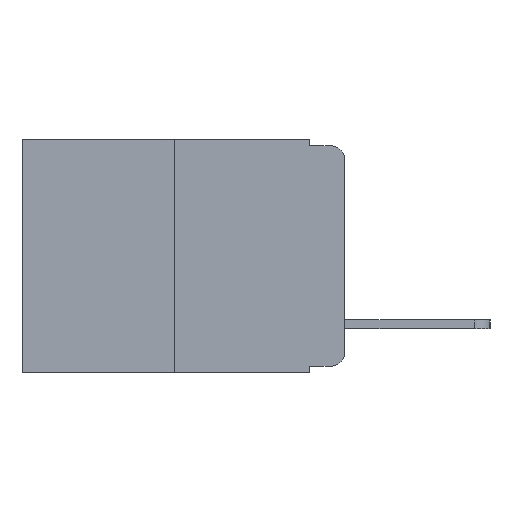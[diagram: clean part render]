
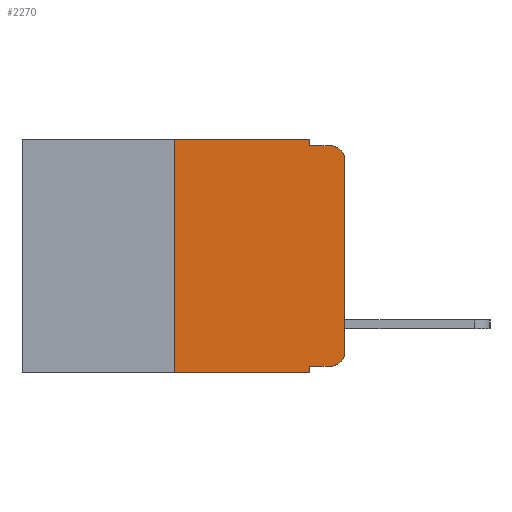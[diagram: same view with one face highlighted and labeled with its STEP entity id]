
A CAD part, left-side view. The second image highlights one B-rep face of the part: STEP entity #2270.
In plain terms, the highlighted planar face has unit normal (-1, 0, 0).
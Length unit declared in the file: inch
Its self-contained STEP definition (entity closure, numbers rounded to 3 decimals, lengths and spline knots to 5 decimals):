
#730 = AXIS2_PLACEMENT_3D ( 'NONE', #4865, #1582, #7941 ) ;
#749 = CARTESIAN_POINT ( 'NONE',  ( 0., 0., -0.03 ) ) ;
#792 = ORIENTED_EDGE ( 'NONE', *, *, #5768, .T. ) ;
#857 = CARTESIAN_POINT ( 'NONE',  ( 0., 0.051, -0.333 ) ) ;
#1050 = ORIENTED_EDGE ( 'NONE', *, *, #5008, .T. ) ;
#1187 = LINE ( 'NONE', #3296, #5474 ) ;
#1582 = DIRECTION ( 'NONE',  ( -1., 0., 0. ) ) ;
#1626 = CARTESIAN_POINT ( 'NONE',  ( 0., 0.25, 0. ) ) ;
#1706 = DIRECTION ( 'NONE',  ( 0., 0., -1. ) ) ;
#1768 = DIRECTION ( 'NONE',  ( 0., 0., -1. ) ) ;
#1894 = CIRCLE ( 'NONE', #2462, 0.02 ) ;
#1895 = CARTESIAN_POINT ( 'NONE',  ( 0., 0.25, 0. ) ) ;
#2013 = ORIENTED_EDGE ( 'NONE', *, *, #5486, .F. ) ;
#2041 = CARTESIAN_POINT ( 'NONE',  ( 0., 0.051, -0.01 ) ) ;
#2056 = VECTOR ( 'NONE', #8655, 39.37008 ) ;
#2193 = VERTEX_POINT ( 'NONE', #9770 ) ;
#2208 = VECTOR ( 'NONE', #6875, 39.37008 ) ;
#2270 = ADVANCED_FACE ( 'NONE', ( #4684 ), #4463, .F. ) ;
#2276 = VERTEX_POINT ( 'NONE', #5153 ) ;
#2317 = ORIENTED_EDGE ( 'NONE', *, *, #5647, .F. ) ;
#2462 = AXIS2_PLACEMENT_3D ( 'NONE', #5428, #5593, #1768 ) ;
#2519 = LINE ( 'NONE', #9685, #8420 ) ;
#2572 = DIRECTION ( 'NONE',  ( 0., -1., 0. ) ) ;
#2662 = EDGE_CURVE ( 'NONE', #4297, #4433, #1187, .T. ) ;
#2743 = CARTESIAN_POINT ( 'NONE',  ( 0., 0., 0. ) ) ;
#2974 = VECTOR ( 'NONE', #2572, 39.37008 ) ;
#3042 = DIRECTION ( 'NONE',  ( 0., 0., 1. ) ) ;
#3130 = CIRCLE ( 'NONE', #730, 0.02 ) ;
#3169 = AXIS2_PLACEMENT_3D ( 'NONE', #5853, #4576, #4569 ) ;
#3296 = CARTESIAN_POINT ( 'NONE',  ( 0., 0.473, -0.343 ) ) ;
#3309 = DIRECTION ( 'NONE',  ( 0., -1., 0. ) ) ;
#3364 = CARTESIAN_POINT ( 'NONE',  ( 0., 0.051, -0.333 ) ) ;
#3381 = ORIENTED_EDGE ( 'NONE', *, *, #5251, .F. ) ;
#4239 = VERTEX_POINT ( 'NONE', #1895 ) ;
#4297 = VERTEX_POINT ( 'NONE', #7303 ) ;
#4299 = LINE ( 'NONE', #6160, #6185 ) ;
#4433 = VERTEX_POINT ( 'NONE', #5621 ) ;
#4463 = PLANE ( 'NONE',  #3169 ) ;
#4569 = DIRECTION ( 'NONE',  ( 0., 0., -1. ) ) ;
#4576 = DIRECTION ( 'NONE',  ( 1., 0., 0. ) ) ;
#4588 = LINE ( 'NONE', #3364, #2208 ) ;
#4623 = CARTESIAN_POINT ( 'NONE',  ( 0., 0.02, -0.333 ) ) ;
#4684 = FACE_OUTER_BOUND ( 'NONE', #5697, .T. ) ;
#4700 = LINE ( 'NONE', #9311, #2056 ) ;
#4778 = DIRECTION ( 'NONE',  ( 0., -1., 0. ) ) ;
#4865 = CARTESIAN_POINT ( 'NONE',  ( 0., 0.02, -0.03 ) ) ;
#5008 = EDGE_CURVE ( 'NONE', #2276, #9101, #6620, .T. ) ;
#5024 = ORIENTED_EDGE ( 'NONE', *, *, #5137, .T. ) ;
#5086 = VERTEX_POINT ( 'NONE', #857 ) ;
#5137 = EDGE_CURVE ( 'NONE', #9101, #9544, #3130, .T. ) ;
#5153 = CARTESIAN_POINT ( 'NONE',  ( 0., 0., -0.313 ) ) ;
#5251 = EDGE_CURVE ( 'NONE', #5674, #9544, #7285, .T. ) ;
#5295 = LINE ( 'NONE', #1626, #6934 ) ;
#5322 = EDGE_CURVE ( 'NONE', #2193, #5674, #4700, .T. ) ;
#5323 = CARTESIAN_POINT ( 'NONE',  ( 0., 0.051, -0.01 ) ) ;
#5428 = CARTESIAN_POINT ( 'NONE',  ( 0., 0.02, -0.313 ) ) ;
#5474 = VECTOR ( 'NONE', #3309, 39.37008 ) ;
#5486 = EDGE_CURVE ( 'NONE', #4297, #4239, #5295, .T. ) ;
#5593 = DIRECTION ( 'NONE',  ( -1., 0., 0. ) ) ;
#5621 = CARTESIAN_POINT ( 'NONE',  ( 0., 0.051, -0.343 ) ) ;
#5647 = EDGE_CURVE ( 'NONE', #5086, #4433, #2519, .T. ) ;
#5674 = VERTEX_POINT ( 'NONE', #5323 ) ;
#5697 = EDGE_LOOP ( 'NONE', ( #1050, #5024, #3381, #7355, #5888, #2013, #8284, #2317, #8948, #792 ) ) ;
#5703 = EDGE_CURVE ( 'NONE', #5086, #5995, #4588, .T. ) ;
#5768 = EDGE_CURVE ( 'NONE', #5995, #2276, #1894, .T. ) ;
#5853 = CARTESIAN_POINT ( 'NONE',  ( 0., 0.473, 0. ) ) ;
#5888 = ORIENTED_EDGE ( 'NONE', *, *, #9551, .F. ) ;
#5995 = VERTEX_POINT ( 'NONE', #4623 ) ;
#6160 = CARTESIAN_POINT ( 'NONE',  ( 0., 0.473, 0. ) ) ;
#6185 = VECTOR ( 'NONE', #4778, 39.37008 ) ;
#6620 = LINE ( 'NONE', #2743, #9951 ) ;
#6875 = DIRECTION ( 'NONE',  ( 0., -1., 0. ) ) ;
#6934 = VECTOR ( 'NONE', #3042, 39.37008 ) ;
#7285 = LINE ( 'NONE', #2041, #2974 ) ;
#7303 = CARTESIAN_POINT ( 'NONE',  ( 0., 0.25, -0.343 ) ) ;
#7355 = ORIENTED_EDGE ( 'NONE', *, *, #5322, .F. ) ;
#7941 = DIRECTION ( 'NONE',  ( 0., 0., -1. ) ) ;
#8284 = ORIENTED_EDGE ( 'NONE', *, *, #2662, .T. ) ;
#8420 = VECTOR ( 'NONE', #1706, 39.37008 ) ;
#8655 = DIRECTION ( 'NONE',  ( 0., 0., -1. ) ) ;
#8732 = DIRECTION ( 'NONE',  ( 0., 0., 1. ) ) ;
#8948 = ORIENTED_EDGE ( 'NONE', *, *, #5703, .T. ) ;
#9101 = VERTEX_POINT ( 'NONE', #749 ) ;
#9311 = CARTESIAN_POINT ( 'NONE',  ( 0., 0.051, 0. ) ) ;
#9544 = VERTEX_POINT ( 'NONE', #9733 ) ;
#9551 = EDGE_CURVE ( 'NONE', #4239, #2193, #4299, .T. ) ;
#9685 = CARTESIAN_POINT ( 'NONE',  ( 0., 0.051, 0. ) ) ;
#9733 = CARTESIAN_POINT ( 'NONE',  ( 0., 0.02, -0.01 ) ) ;
#9770 = CARTESIAN_POINT ( 'NONE',  ( 0., 0.051, 0. ) ) ;
#9951 = VECTOR ( 'NONE', #8732, 39.37008 ) ;
